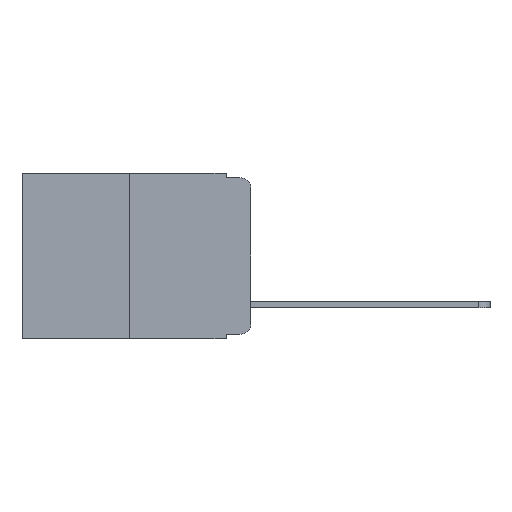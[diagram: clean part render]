
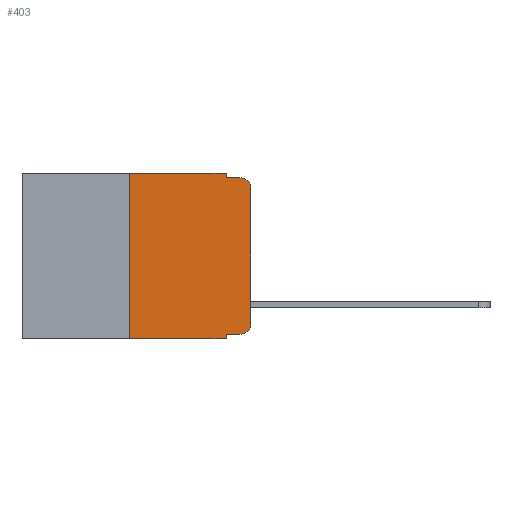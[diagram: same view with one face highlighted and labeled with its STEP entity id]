
A CAD part, left-side view. The second image highlights one B-rep face of the part: STEP entity #403.
In plain terms, the highlighted planar face has unit normal (-1, 0, 0).
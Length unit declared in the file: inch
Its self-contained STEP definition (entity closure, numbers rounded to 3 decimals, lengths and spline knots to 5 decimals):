
#116 = PLANE ( 'NONE',  #4852 ) ;
#154 = VERTEX_POINT ( 'NONE', #13122 ) ;
#220 = DIRECTION ( 'NONE',  ( 0., 0., -1. ) ) ;
#278 = CARTESIAN_POINT ( 'NONE',  ( 0., 0.473, 0. ) ) ;
#296 = EDGE_LOOP ( 'NONE', ( #1928, #14135, #1607, #10838, #14425, #405, #4918, #13407, #4932, #9026 ) ) ;
#403 = ADVANCED_FACE ( 'NONE', ( #13431 ), #116, .F. ) ;
#405 = ORIENTED_EDGE ( 'NONE', *, *, #6485, .F. ) ;
#764 = CARTESIAN_POINT ( 'NONE',  ( 0., 0.051, 0. ) ) ;
#1093 = CARTESIAN_POINT ( 'NONE',  ( 0., 0.473, 0. ) ) ;
#1415 = EDGE_CURVE ( 'NONE', #13472, #10365, #5572, .T. ) ;
#1607 = ORIENTED_EDGE ( 'NONE', *, *, #15208, .F. ) ;
#1724 = EDGE_CURVE ( 'NONE', #10287, #154, #9648, .T. ) ;
#1826 = EDGE_CURVE ( 'NONE', #10287, #14755, #9254, .T. ) ;
#1928 = ORIENTED_EDGE ( 'NONE', *, *, #10234, .T. ) ;
#1974 = CARTESIAN_POINT ( 'NONE',  ( 0., 0.051, -0.01 ) ) ;
#1993 = DIRECTION ( 'NONE',  ( 0., 0., -1. ) ) ;
#2478 = DIRECTION ( 'NONE',  ( -1., 0., 0. ) ) ;
#2540 = VERTEX_POINT ( 'NONE', #7878 ) ;
#3192 = CARTESIAN_POINT ( 'NONE',  ( 0., 0.25, -0.343 ) ) ;
#3194 = VECTOR ( 'NONE', #10421, 39.37008 ) ;
#3587 = VECTOR ( 'NONE', #16005, 39.37008 ) ;
#3658 = CARTESIAN_POINT ( 'NONE',  ( 0., 0., 0. ) ) ;
#3682 = CARTESIAN_POINT ( 'NONE',  ( 0., 0.02, -0.03 ) ) ;
#4133 = CARTESIAN_POINT ( 'NONE',  ( 0., 0.051, -0.01 ) ) ;
#4852 = AXIS2_PLACEMENT_3D ( 'NONE', #278, #8896, #220 ) ;
#4918 = ORIENTED_EDGE ( 'NONE', *, *, #13230, .T. ) ;
#4932 = ORIENTED_EDGE ( 'NONE', *, *, #1724, .T. ) ;
#5473 = VERTEX_POINT ( 'NONE', #11923 ) ;
#5572 = CIRCLE ( 'NONE', #16014, 0.02 ) ;
#5659 = VECTOR ( 'NONE', #13500, 39.37008 ) ;
#6119 = EDGE_CURVE ( 'NONE', #11280, #9024, #11114, .T. ) ;
#6307 = CARTESIAN_POINT ( 'NONE',  ( 0., 0.051, -0.343 ) ) ;
#6485 = EDGE_CURVE ( 'NONE', #15418, #5473, #14045, .T. ) ;
#6911 = DIRECTION ( 'NONE',  ( 0., 0., -1. ) ) ;
#6970 = CARTESIAN_POINT ( 'NONE',  ( 0., 0.051, 0. ) ) ;
#7120 = VECTOR ( 'NONE', #1993, 39.37008 ) ;
#7279 = CARTESIAN_POINT ( 'NONE',  ( 0., 0.051, -0.333 ) ) ;
#7799 = VECTOR ( 'NONE', #6911, 39.37008 ) ;
#7878 = CARTESIAN_POINT ( 'NONE',  ( 0., 0., -0.313 ) ) ;
#8107 = DIRECTION ( 'NONE',  ( 0., -1., 0. ) ) ;
#8279 = EDGE_CURVE ( 'NONE', #5473, #11280, #12724, .T. ) ;
#8459 = LINE ( 'NONE', #3658, #10028 ) ;
#8470 = VECTOR ( 'NONE', #8107, 39.37008 ) ;
#8896 = DIRECTION ( 'NONE',  ( 1., 0., 0. ) ) ;
#8977 = DIRECTION ( 'NONE',  ( -1., 0., 0. ) ) ;
#9024 = VERTEX_POINT ( 'NONE', #1974 ) ;
#9026 = ORIENTED_EDGE ( 'NONE', *, *, #12722, .T. ) ;
#9254 = LINE ( 'NONE', #6970, #7120 ) ;
#9648 = LINE ( 'NONE', #13076, #8470 ) ;
#9897 = DIRECTION ( 'NONE',  ( 0., 0., 1. ) ) ;
#10028 = VECTOR ( 'NONE', #9897, 39.37008 ) ;
#10234 = EDGE_CURVE ( 'NONE', #2540, #13472, #8459, .T. ) ;
#10287 = VERTEX_POINT ( 'NONE', #7279 ) ;
#10365 = VERTEX_POINT ( 'NONE', #12622 ) ;
#10421 = DIRECTION ( 'NONE',  ( 0., -1., 0. ) ) ;
#10579 = VECTOR ( 'NONE', #13378, 39.37008 ) ;
#10838 = ORIENTED_EDGE ( 'NONE', *, *, #6119, .F. ) ;
#11114 = LINE ( 'NONE', #11916, #7799 ) ;
#11280 = VERTEX_POINT ( 'NONE', #764 ) ;
#11372 = CARTESIAN_POINT ( 'NONE',  ( 0., 0.02, -0.313 ) ) ;
#11916 = CARTESIAN_POINT ( 'NONE',  ( 0., 0.051, 0. ) ) ;
#11923 = CARTESIAN_POINT ( 'NONE',  ( 0., 0.25, 0. ) ) ;
#12184 = LINE ( 'NONE', #4133, #3194 ) ;
#12467 = DIRECTION ( 'NONE',  ( 0., 0., -1. ) ) ;
#12622 = CARTESIAN_POINT ( 'NONE',  ( 0., 0.02, -0.01 ) ) ;
#12697 = DIRECTION ( 'NONE',  ( 0., 0., -1. ) ) ;
#12722 = EDGE_CURVE ( 'NONE', #154, #2540, #13288, .T. ) ;
#12724 = LINE ( 'NONE', #1093, #10579 ) ;
#13076 = CARTESIAN_POINT ( 'NONE',  ( 0., 0.051, -0.333 ) ) ;
#13122 = CARTESIAN_POINT ( 'NONE',  ( 0., 0.02, -0.333 ) ) ;
#13230 = EDGE_CURVE ( 'NONE', #15418, #14755, #13563, .T. ) ;
#13288 = CIRCLE ( 'NONE', #13710, 0.02 ) ;
#13378 = DIRECTION ( 'NONE',  ( 0., -1., 0. ) ) ;
#13407 = ORIENTED_EDGE ( 'NONE', *, *, #1826, .F. ) ;
#13431 = FACE_OUTER_BOUND ( 'NONE', #296, .T. ) ;
#13464 = CARTESIAN_POINT ( 'NONE',  ( 0., 0.473, -0.343 ) ) ;
#13472 = VERTEX_POINT ( 'NONE', #13882 ) ;
#13500 = DIRECTION ( 'NONE',  ( 0., 0., 1. ) ) ;
#13563 = LINE ( 'NONE', #13464, #3587 ) ;
#13710 = AXIS2_PLACEMENT_3D ( 'NONE', #11372, #8977, #12697 ) ;
#13882 = CARTESIAN_POINT ( 'NONE',  ( 0., 0., -0.03 ) ) ;
#14045 = LINE ( 'NONE', #14806, #5659 ) ;
#14135 = ORIENTED_EDGE ( 'NONE', *, *, #1415, .T. ) ;
#14425 = ORIENTED_EDGE ( 'NONE', *, *, #8279, .F. ) ;
#14755 = VERTEX_POINT ( 'NONE', #6307 ) ;
#14806 = CARTESIAN_POINT ( 'NONE',  ( 0., 0.25, 0. ) ) ;
#15208 = EDGE_CURVE ( 'NONE', #9024, #10365, #12184, .T. ) ;
#15418 = VERTEX_POINT ( 'NONE', #3192 ) ;
#16005 = DIRECTION ( 'NONE',  ( 0., -1., 0. ) ) ;
#16014 = AXIS2_PLACEMENT_3D ( 'NONE', #3682, #2478, #12467 ) ;
